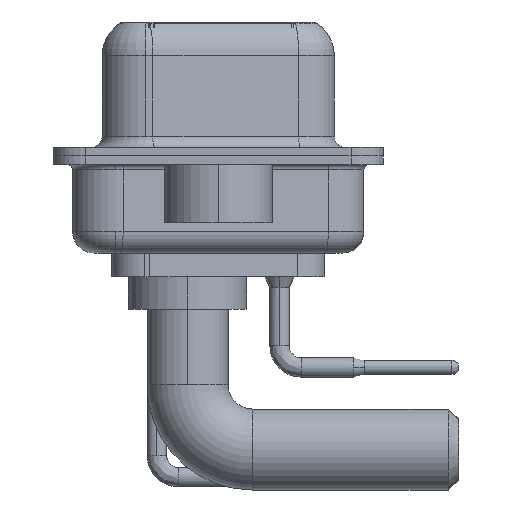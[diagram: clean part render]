
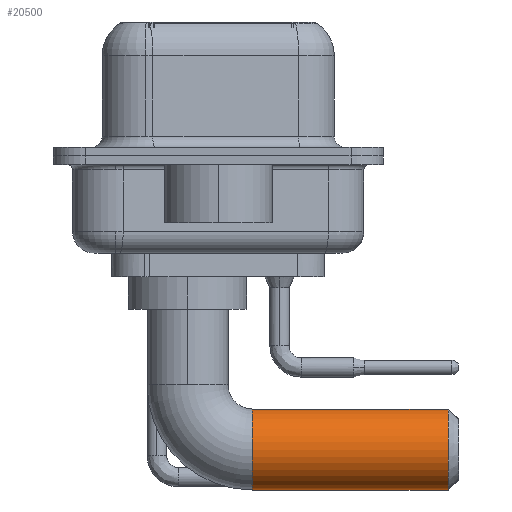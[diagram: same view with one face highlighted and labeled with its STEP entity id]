
A CAD part, left-side view. The second image highlights one B-rep face of the part: STEP entity #20500.
In plain terms, the highlighted cylindrical face has radius 1.875 mm (diameter 3.75 mm), a partial arc.
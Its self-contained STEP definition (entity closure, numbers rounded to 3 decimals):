
#428 = DIRECTION ( 'NONE',  ( 0., -1., 0. ) ) ;
#932 = EDGE_CURVE ( 'NONE', #5156, #24145, #26560, .T. ) ;
#1635 = CARTESIAN_POINT ( 'NONE',  ( 0., -12.07, -4.625 ) ) ;
#3204 = EDGE_LOOP ( 'NONE', ( #4606, #9738, #18765, #20284 ) ) ;
#4606 = ORIENTED_EDGE ( 'NONE', *, *, #26281, .F. ) ;
#5040 = LINE ( 'NONE', #27407, #22599 ) ;
#5156 = VERTEX_POINT ( 'NONE', #8945 ) ;
#5304 = FACE_OUTER_BOUND ( 'NONE', #3204, .T. ) ;
#6266 = DIRECTION ( 'NONE',  ( 0., 0., -1. ) ) ;
#8264 = VERTEX_POINT ( 'NONE', #1635 ) ;
#8945 = CARTESIAN_POINT ( 'NONE',  ( 0., -3., -4.625 ) ) ;
#9423 = VECTOR ( 'NONE', #12803, 1000. ) ;
#9738 = ORIENTED_EDGE ( 'NONE', *, *, #932, .T. ) ;
#9907 = CYLINDRICAL_SURFACE ( 'NONE', #21638, 1.875 ) ;
#10325 = VERTEX_POINT ( 'NONE', #16374 ) ;
#10587 = EDGE_CURVE ( 'NONE', #24145, #10325, #21980, .T. ) ;
#10913 = CIRCLE ( 'NONE', #14199, 1.875 ) ;
#11676 = CARTESIAN_POINT ( 'NONE',  ( 0., -3., -6.5 ) ) ;
#12803 = DIRECTION ( 'NONE',  ( 0., -1., 0. ) ) ;
#14199 = AXIS2_PLACEMENT_3D ( 'NONE', #28787, #17359, #6266 ) ;
#14318 = CARTESIAN_POINT ( 'NONE',  ( 0., -3., -6.5 ) ) ;
#15655 = AXIS2_PLACEMENT_3D ( 'NONE', #11676, #428, #17950 ) ;
#16374 = CARTESIAN_POINT ( 'NONE',  ( 0., -12.07, -8.375 ) ) ;
#16889 = CARTESIAN_POINT ( 'NONE',  ( 0., -3., -8.375 ) ) ;
#17359 = DIRECTION ( 'NONE',  ( 0., 1., 0. ) ) ;
#17950 = DIRECTION ( 'NONE',  ( -1., 0., 0. ) ) ;
#18765 = ORIENTED_EDGE ( 'NONE', *, *, #10587, .T. ) ;
#18910 = DIRECTION ( 'NONE',  ( 0., 0., -1. ) ) ;
#20284 = ORIENTED_EDGE ( 'NONE', *, *, #28611, .T. ) ;
#20500 = ADVANCED_FACE ( 'NONE', ( #5304 ), #9907, .T. ) ;
#21638 = AXIS2_PLACEMENT_3D ( 'NONE', #14318, #23072, #18910 ) ;
#21980 = LINE ( 'NONE', #26882, #9423 ) ;
#22599 = VECTOR ( 'NONE', #23098, 1000. ) ;
#23072 = DIRECTION ( 'NONE',  ( 0., -1., 0. ) ) ;
#23098 = DIRECTION ( 'NONE',  ( 0., -1., 0. ) ) ;
#24145 = VERTEX_POINT ( 'NONE', #16889 ) ;
#26281 = EDGE_CURVE ( 'NONE', #5156, #8264, #5040, .T. ) ;
#26560 = CIRCLE ( 'NONE', #15655, 1.875 ) ;
#26882 = CARTESIAN_POINT ( 'NONE',  ( 0., -3., -8.375 ) ) ;
#27407 = CARTESIAN_POINT ( 'NONE',  ( 0., -3., -4.625 ) ) ;
#28611 = EDGE_CURVE ( 'NONE', #10325, #8264, #10913, .T. ) ;
#28787 = CARTESIAN_POINT ( 'NONE',  ( 0., -12.07, -6.5 ) ) ;
